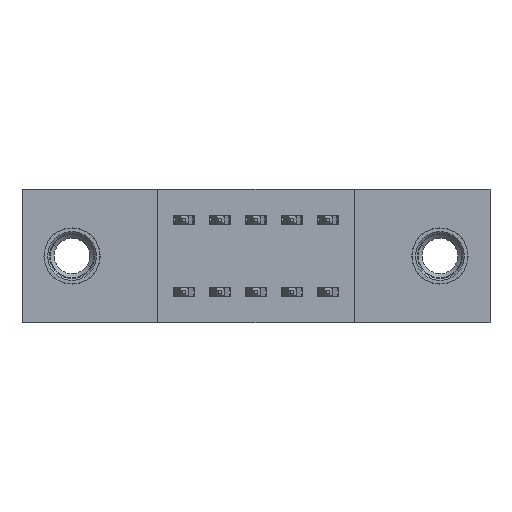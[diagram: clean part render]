
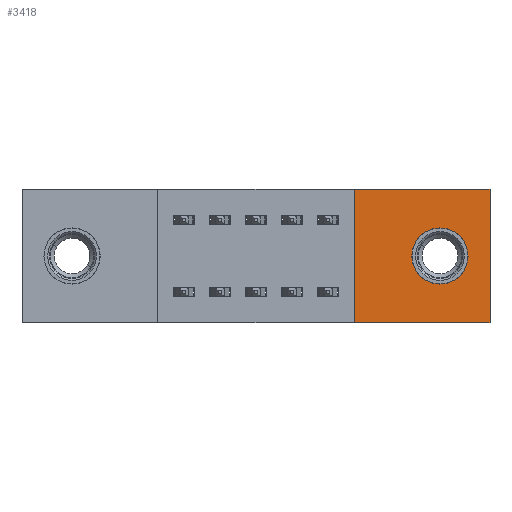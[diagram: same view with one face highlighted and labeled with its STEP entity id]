
A CAD part, front view. The second image highlights one B-rep face of the part: STEP entity #3418.
In plain terms, the highlighted planar face has unit normal (0, -1, 0).
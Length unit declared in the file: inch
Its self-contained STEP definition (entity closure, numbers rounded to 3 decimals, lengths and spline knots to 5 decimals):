
#54 = VECTOR ( 'NONE', #880, 39.37008 ) ;
#505 = CARTESIAN_POINT ( 'NONE',  ( 1.161, 0., -0.107 ) ) ;
#740 = CIRCLE ( 'NONE', #6746, 0.078 ) ;
#880 = DIRECTION ( 'NONE',  ( 1., 0., 0. ) ) ;
#1153 = LINE ( 'NONE', #2117, #4805 ) ;
#1183 = AXIS2_PLACEMENT_3D ( 'NONE', #7970, #3851, #8645 ) ;
#1409 = CARTESIAN_POINT ( 'NONE',  ( 1.3, 0., 0. ) ) ;
#1486 = ORIENTED_EDGE ( 'NONE', *, *, #7529, .F. ) ;
#1648 = AXIS2_PLACEMENT_3D ( 'NONE', #8677, #8438, #8426 ) ;
#1911 = DIRECTION ( 'NONE',  ( -1., 0., 0. ) ) ;
#2068 = CARTESIAN_POINT ( 'NONE',  ( 1.161, 0., -0.185 ) ) ;
#2117 = CARTESIAN_POINT ( 'NONE',  ( 0.923, 0., -0.37 ) ) ;
#2446 = EDGE_LOOP ( 'NONE', ( #1486, #5704, #6889, #3634 ) ) ;
#2776 = ORIENTED_EDGE ( 'NONE', *, *, #5721, .T. ) ;
#2809 = DIRECTION ( 'NONE',  ( 0., 0., -1. ) ) ;
#2958 = FACE_BOUND ( 'NONE', #5310, .T. ) ;
#3237 = VECTOR ( 'NONE', #1911, 39.37008 ) ;
#3384 = ORIENTED_EDGE ( 'NONE', *, *, #6095, .T. ) ;
#3418 = ADVANCED_FACE ( 'NONE', ( #2958, #5112 ), #8493, .T. ) ;
#3634 = ORIENTED_EDGE ( 'NONE', *, *, #5691, .F. ) ;
#3851 = DIRECTION ( 'NONE',  ( 0., 1., 0. ) ) ;
#4332 = DIRECTION ( 'NONE',  ( 0., 0., 1. ) ) ;
#4514 = CARTESIAN_POINT ( 'NONE',  ( 0.923, 0., 0. ) ) ;
#4521 = CARTESIAN_POINT ( 'NONE',  ( 0., 0., 0. ) ) ;
#4549 = VERTEX_POINT ( 'NONE', #5836 ) ;
#4805 = VECTOR ( 'NONE', #4332, 39.37008 ) ;
#4938 = CARTESIAN_POINT ( 'NONE',  ( 1.3, 0., 0. ) ) ;
#5112 = FACE_OUTER_BOUND ( 'NONE', #2446, .T. ) ;
#5264 = VERTEX_POINT ( 'NONE', #6797 ) ;
#5310 = EDGE_LOOP ( 'NONE', ( #2776, #3384 ) ) ;
#5571 = VECTOR ( 'NONE', #7620, 39.37008 ) ;
#5691 = EDGE_CURVE ( 'NONE', #6311, #7558, #5813, .T. ) ;
#5704 = ORIENTED_EDGE ( 'NONE', *, *, #7992, .F. ) ;
#5721 = EDGE_CURVE ( 'NONE', #9070, #4549, #7391, .T. ) ;
#5813 = LINE ( 'NONE', #4521, #54 ) ;
#5836 = CARTESIAN_POINT ( 'NONE',  ( 1.161, 0., -0.263 ) ) ;
#5949 = VERTEX_POINT ( 'NONE', #8201 ) ;
#6095 = EDGE_CURVE ( 'NONE', #4549, #9070, #740, .T. ) ;
#6197 = CARTESIAN_POINT ( 'NONE',  ( 0., 0., -0.37 ) ) ;
#6311 = VERTEX_POINT ( 'NONE', #4514 ) ;
#6746 = AXIS2_PLACEMENT_3D ( 'NONE', #2068, #7005, #2809 ) ;
#6797 = CARTESIAN_POINT ( 'NONE',  ( 0.923, 0., -0.37 ) ) ;
#6889 = ORIENTED_EDGE ( 'NONE', *, *, #8439, .F. ) ;
#7005 = DIRECTION ( 'NONE',  ( 0., 1., 0. ) ) ;
#7391 = CIRCLE ( 'NONE', #1183, 0.078 ) ;
#7529 = EDGE_CURVE ( 'NONE', #5264, #6311, #1153, .T. ) ;
#7558 = VERTEX_POINT ( 'NONE', #1409 ) ;
#7620 = DIRECTION ( 'NONE',  ( 0., 0., -1. ) ) ;
#7970 = CARTESIAN_POINT ( 'NONE',  ( 1.161, 0., -0.185 ) ) ;
#7992 = EDGE_CURVE ( 'NONE', #5949, #5264, #8521, .T. ) ;
#7999 = LINE ( 'NONE', #4938, #5571 ) ;
#8201 = CARTESIAN_POINT ( 'NONE',  ( 1.3, 0., -0.37 ) ) ;
#8426 = DIRECTION ( 'NONE',  ( 0., 0., -1. ) ) ;
#8438 = DIRECTION ( 'NONE',  ( 0., -1., 0. ) ) ;
#8439 = EDGE_CURVE ( 'NONE', #7558, #5949, #7999, .T. ) ;
#8493 = PLANE ( 'NONE',  #1648 ) ;
#8521 = LINE ( 'NONE', #6197, #3237 ) ;
#8645 = DIRECTION ( 'NONE',  ( 0., 0., -1. ) ) ;
#8677 = CARTESIAN_POINT ( 'NONE',  ( 0., 0., -0.37 ) ) ;
#9070 = VERTEX_POINT ( 'NONE', #505 ) ;
